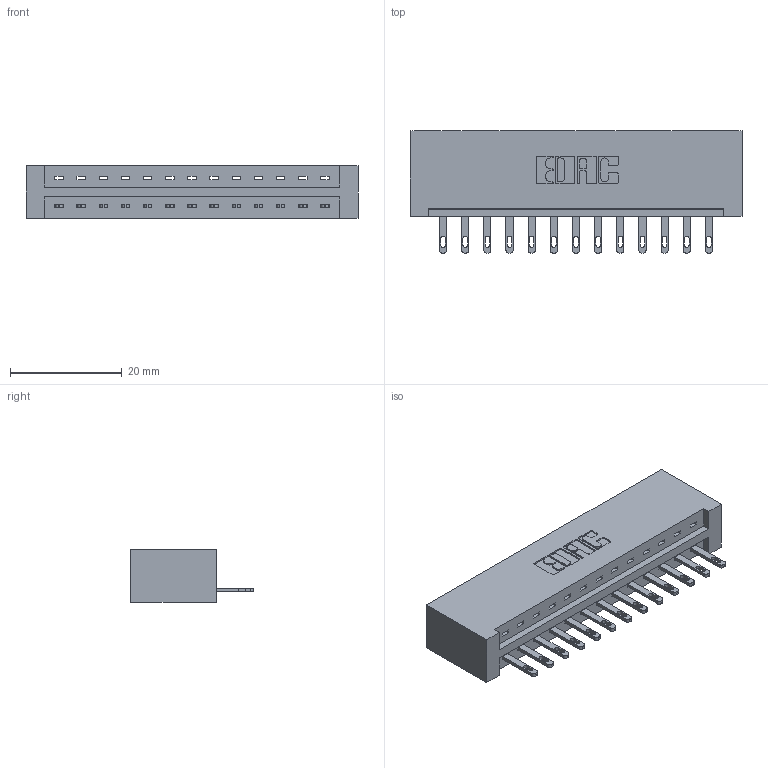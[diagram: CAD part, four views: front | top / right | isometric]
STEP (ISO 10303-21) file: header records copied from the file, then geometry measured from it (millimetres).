
FILE_DESCRIPTION (( 'STEP AP203' ), '1' );
FILE_NAME ('887-013-500-101.STEP', '2020-09-20T16:32:47', ( '' ), ( '' ), 'SwSTEP 2.0', 'SolidWorks 2020', '' );
FILE_SCHEMA (( 'CONFIG_CONTROL_DESIGN' ));
Length unit declared in the file: inch
Products named in the file (3): 887-013-500-101; 345-292-001_345-293-100; 837 Part_No Mounting Lugs
Assembly tree (14 placements, depth 2):
  887-013-500-101
    837 Part_No Mounting Lugs
    345-292-001_345-293-100  x13
Bounding box: 59.39 x 21.85 x 9.4 mm (x, y, z)
Volume: 6556 mm3; surface area: 6625.4 mm2
Topology: 14 solids, 14 shells, 860 faces, 2627 edges, 1750 vertices
Faces by surface type: plane 586, cylinder 274
Entity records: 13067 total; most frequent: CARTESIAN_POINT 2281, ORIENTED_EDGE 2230, DIRECTION 1973, EDGE_CURVE 1115, LINE 991, VECTOR 991, VERTEX_POINT 742, AXIS2_PLACEMENT_3D 491
